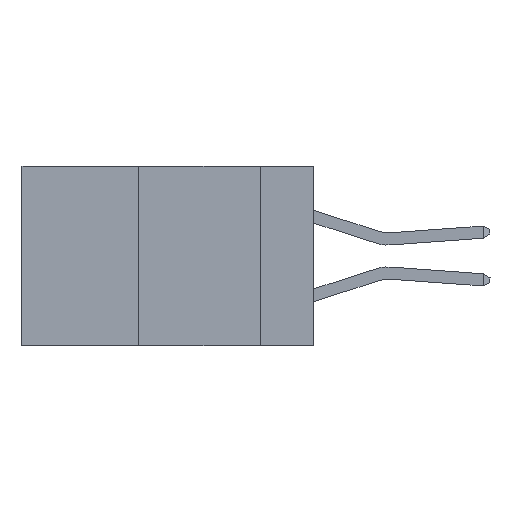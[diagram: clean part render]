
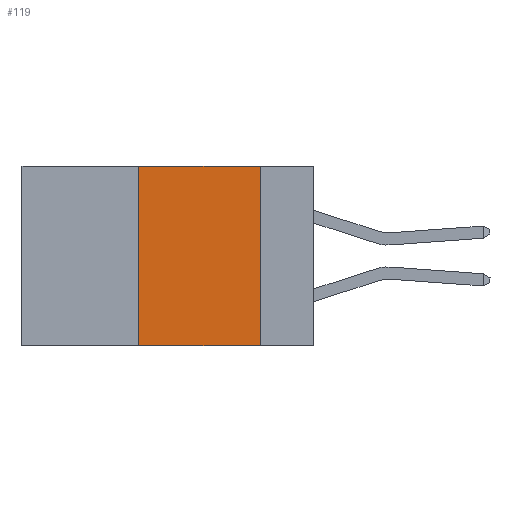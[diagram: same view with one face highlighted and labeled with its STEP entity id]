
A CAD part, left-side view. The second image highlights one B-rep face of the part: STEP entity #119.
In plain terms, the highlighted planar face has unit normal (-1, 0, 0).
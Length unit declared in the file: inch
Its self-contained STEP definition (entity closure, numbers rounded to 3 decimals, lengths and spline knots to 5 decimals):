
#119 = ADVANCED_FACE ( 'NONE', ( #6491 ), #23407, .F. ) ;
#237 = DIRECTION ( 'NONE',  ( 0., 0., 1. ) ) ;
#564 = LINE ( 'NONE', #21222, #4302 ) ;
#1035 = CARTESIAN_POINT ( 'NONE',  ( 0., 0.6, 0. ) ) ;
#2563 = EDGE_CURVE ( 'NONE', #8068, #7707, #564, .T. ) ;
#2925 = LINE ( 'NONE', #7614, #22712 ) ;
#3745 = EDGE_LOOP ( 'NONE', ( #22584, #23736, #6368, #17882 ) ) ;
#4141 = DIRECTION ( 'NONE',  ( 0., 0., -1. ) ) ;
#4302 = VECTOR ( 'NONE', #14133, 39.37008 ) ;
#4922 = CARTESIAN_POINT ( 'NONE',  ( 0., 0.36, -0.37 ) ) ;
#6000 = CARTESIAN_POINT ( 'NONE',  ( 0., 0.36, 0. ) ) ;
#6327 = DIRECTION ( 'NONE',  ( 0., -1., 0. ) ) ;
#6368 = ORIENTED_EDGE ( 'NONE', *, *, #9197, .F. ) ;
#6491 = FACE_OUTER_BOUND ( 'NONE', #3745, .T. ) ;
#6495 = LINE ( 'NONE', #17508, #20834 ) ;
#7614 = CARTESIAN_POINT ( 'NONE',  ( 0., 0.36, 0. ) ) ;
#7707 = VERTEX_POINT ( 'NONE', #17173 ) ;
#7726 = CARTESIAN_POINT ( 'NONE',  ( 0., 0.11, 0. ) ) ;
#8068 = VERTEX_POINT ( 'NONE', #6000 ) ;
#8222 = DIRECTION ( 'NONE',  ( 1., 0., 0. ) ) ;
#9197 = EDGE_CURVE ( 'NONE', #21262, #8068, #2925, .T. ) ;
#11057 = LINE ( 'NONE', #7726, #15726 ) ;
#12208 = EDGE_CURVE ( 'NONE', #21262, #18234, #6495, .T. ) ;
#12221 = DIRECTION ( 'NONE',  ( 0., 0., -1. ) ) ;
#12871 = AXIS2_PLACEMENT_3D ( 'NONE', #1035, #8222, #12221 ) ;
#13006 = CARTESIAN_POINT ( 'NONE',  ( 0., 0.11, -0.37 ) ) ;
#14133 = DIRECTION ( 'NONE',  ( 0., -1., 0. ) ) ;
#15726 = VECTOR ( 'NONE', #4141, 39.37008 ) ;
#17173 = CARTESIAN_POINT ( 'NONE',  ( 0., 0.11, 0. ) ) ;
#17508 = CARTESIAN_POINT ( 'NONE',  ( 0., 0.6, -0.37 ) ) ;
#17882 = ORIENTED_EDGE ( 'NONE', *, *, #12208, .T. ) ;
#18234 = VERTEX_POINT ( 'NONE', #13006 ) ;
#20559 = EDGE_CURVE ( 'NONE', #7707, #18234, #11057, .T. ) ;
#20834 = VECTOR ( 'NONE', #6327, 39.37008 ) ;
#21222 = CARTESIAN_POINT ( 'NONE',  ( 0., 0.6, 0. ) ) ;
#21262 = VERTEX_POINT ( 'NONE', #4922 ) ;
#22584 = ORIENTED_EDGE ( 'NONE', *, *, #20559, .F. ) ;
#22712 = VECTOR ( 'NONE', #237, 39.37008 ) ;
#23407 = PLANE ( 'NONE',  #12871 ) ;
#23736 = ORIENTED_EDGE ( 'NONE', *, *, #2563, .F. ) ;
